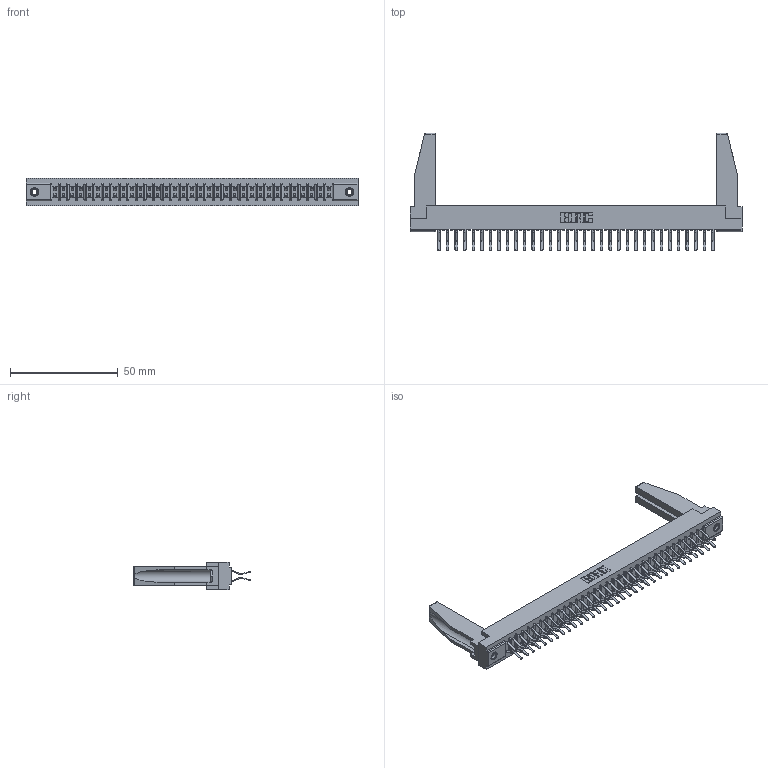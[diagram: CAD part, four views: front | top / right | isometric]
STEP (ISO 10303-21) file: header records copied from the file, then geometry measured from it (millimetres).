
FILE_DESCRIPTION (( 'STEP AP203' ), '1' );
FILE_NAME ('307-066-560-278.STEP', '2019-09-06T18:33:26', ( '' ), ( '' ), 'SwSTEP 2.0', 'SolidWorks 2016', '' );
FILE_SCHEMA (( 'CONFIG_CONTROL_DESIGN' ));
Length unit declared in the file: inch
Products named in the file (5): 307-220-078; 307 Part_.156 Dia Mounting Holes; 307-066-560-278; 345-250-001_345-250-001-102; 307-290-001_560
Assembly tree (71 placements, depth 2):
  307-066-560-278
    307 Part_.156 Dia Mounting Holes
    307-290-001_560  x66
    307-220-078  x2
    345-250-001_345-250-001-102  x2
Bounding box: 153.77 x 54.43 x 12.7 mm (x, y, z)
Volume: 20363.6 mm3; surface area: 24117.8 mm2
Topology: 71 solids, 71 shells, 3582 faces, 10025 edges, 6494 vertices
Faces by surface type: plane 2332, cylinder 1166, sphere 68, cone 12, torus 4
Entity records: 32999 total; most frequent: CARTESIAN_POINT 5411, ORIENTED_EDGE 5320, DIRECTION 5258, EDGE_CURVE 2660, VECTOR 2040, LINE 2040, VERTEX_POINT 1720, AXIS2_PLACEMENT_3D 1609
